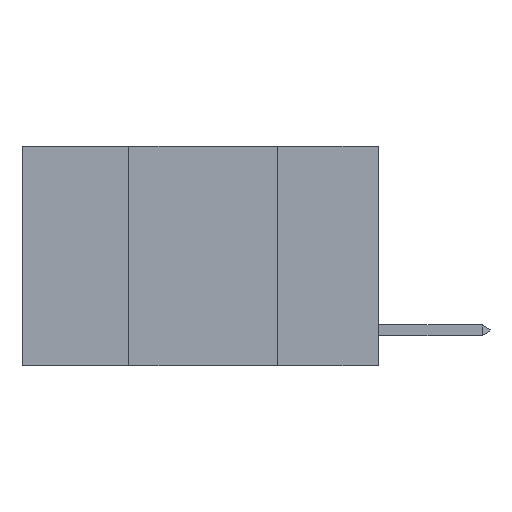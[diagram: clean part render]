
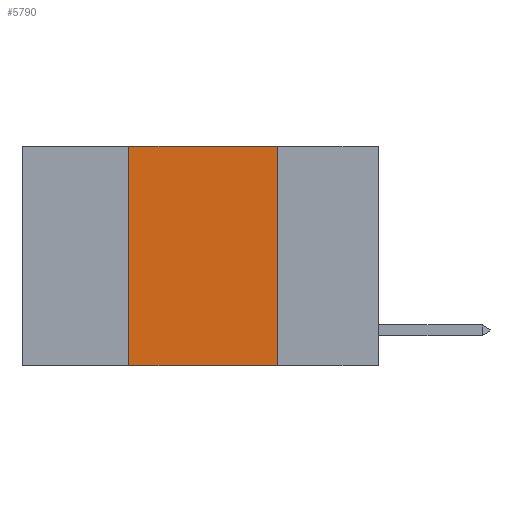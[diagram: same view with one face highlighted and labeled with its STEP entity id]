
A CAD part, left-side view. The second image highlights one B-rep face of the part: STEP entity #5790.
In plain terms, the highlighted planar face has unit normal (-1, 0, 0).
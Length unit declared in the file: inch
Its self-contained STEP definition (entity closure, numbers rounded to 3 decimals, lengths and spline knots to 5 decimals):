
#185 = EDGE_CURVE ( 'NONE', #9632, #16317, #5675, .T. ) ;
#420 = CARTESIAN_POINT ( 'NONE',  ( 0., 0.6, 0. ) ) ;
#673 = PLANE ( 'NONE',  #13660 ) ;
#1888 = LINE ( 'NONE', #9468, #18537 ) ;
#3330 = EDGE_CURVE ( 'NONE', #18102, #7972, #9993, .T. ) ;
#3341 = CARTESIAN_POINT ( 'NONE',  ( 0., 0.42, 0. ) ) ;
#3770 = EDGE_CURVE ( 'NONE', #9632, #18102, #8071, .T. ) ;
#4104 = FACE_OUTER_BOUND ( 'NONE', #9717, .T. ) ;
#5318 = DIRECTION ( 'NONE',  ( 0., 0., -1. ) ) ;
#5491 = VECTOR ( 'NONE', #16564, 39.37008 ) ;
#5675 = LINE ( 'NONE', #18059, #5491 ) ;
#5790 = ADVANCED_FACE ( 'NONE', ( #4104 ), #673, .F. ) ;
#7972 = VERTEX_POINT ( 'NONE', #12188 ) ;
#8004 = DIRECTION ( 'NONE',  ( 0., -1., 0. ) ) ;
#8055 = DIRECTION ( 'NONE',  ( 0., 0., -1. ) ) ;
#8071 = LINE ( 'NONE', #3341, #16188 ) ;
#8921 = ORIENTED_EDGE ( 'NONE', *, *, #3330, .F. ) ;
#9292 = CARTESIAN_POINT ( 'NONE',  ( 0., 0.42, 0. ) ) ;
#9452 = ORIENTED_EDGE ( 'NONE', *, *, #11687, .F. ) ;
#9468 = CARTESIAN_POINT ( 'NONE',  ( 0., 0.17, 0. ) ) ;
#9481 = DIRECTION ( 'NONE',  ( 0., 0., 1. ) ) ;
#9632 = VERTEX_POINT ( 'NONE', #18984 ) ;
#9717 = EDGE_LOOP ( 'NONE', ( #9452, #8921, #18664, #19543 ) ) ;
#9993 = LINE ( 'NONE', #420, #10079 ) ;
#10079 = VECTOR ( 'NONE', #8004, 39.37008 ) ;
#10137 = CARTESIAN_POINT ( 'NONE',  ( 0., 0.6, 0. ) ) ;
#11687 = EDGE_CURVE ( 'NONE', #7972, #16317, #1888, .T. ) ;
#12188 = CARTESIAN_POINT ( 'NONE',  ( 0., 0.17, 0. ) ) ;
#13507 = CARTESIAN_POINT ( 'NONE',  ( 0., 0.17, -0.37 ) ) ;
#13660 = AXIS2_PLACEMENT_3D ( 'NONE', #10137, #19324, #5318 ) ;
#16188 = VECTOR ( 'NONE', #9481, 39.37008 ) ;
#16317 = VERTEX_POINT ( 'NONE', #13507 ) ;
#16564 = DIRECTION ( 'NONE',  ( 0., -1., 0. ) ) ;
#18059 = CARTESIAN_POINT ( 'NONE',  ( 0., 0.6, -0.37 ) ) ;
#18102 = VERTEX_POINT ( 'NONE', #9292 ) ;
#18537 = VECTOR ( 'NONE', #8055, 39.37008 ) ;
#18664 = ORIENTED_EDGE ( 'NONE', *, *, #3770, .F. ) ;
#18984 = CARTESIAN_POINT ( 'NONE',  ( 0., 0.42, -0.37 ) ) ;
#19324 = DIRECTION ( 'NONE',  ( 1., 0., 0. ) ) ;
#19543 = ORIENTED_EDGE ( 'NONE', *, *, #185, .T. ) ;
